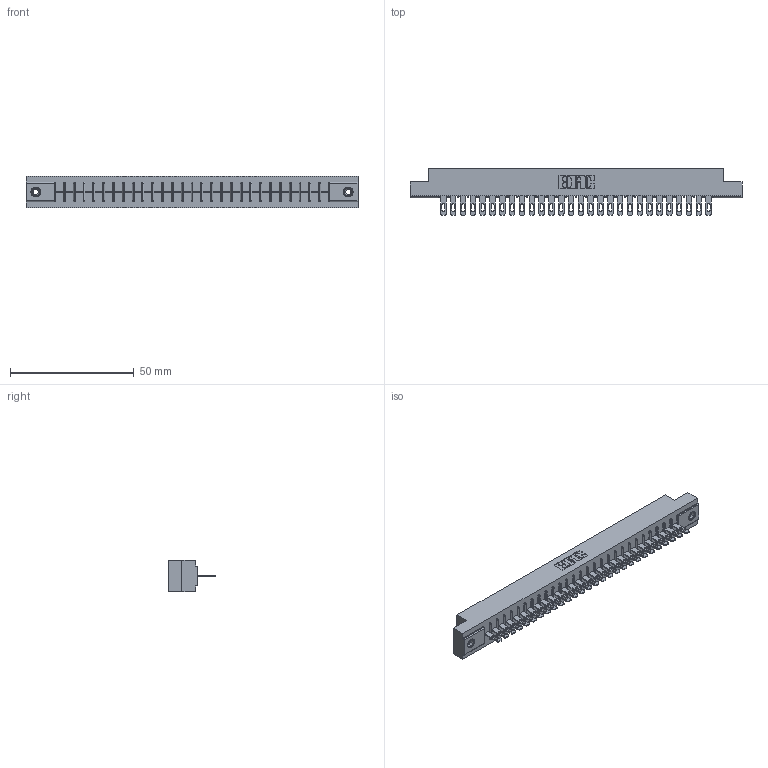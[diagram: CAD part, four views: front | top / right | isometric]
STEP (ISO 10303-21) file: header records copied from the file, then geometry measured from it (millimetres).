
FILE_DESCRIPTION (( 'STEP AP203' ), '1' );
FILE_NAME ('316-028-400-108.STEP', '2020-09-22T23:19:40', ( '' ), ( '' ), 'SwSTEP 2.0', 'SolidWorks 2020', '' );
FILE_SCHEMA (( 'CONFIG_CONTROL_DESIGN' ));
Length unit declared in the file: inch
Products named in the file (4): 345-250-001_345-250-003-102; 306-290-001_100; 316-028-400-108; 306 Part_.156 Dia
Assembly tree (31 placements, depth 2):
  316-028-400-108
    306 Part_.156 Dia
    306-290-001_100  x28
    345-250-001_345-250-003-102  x2
Bounding box: 133.96 x 18.87 x 12.7 mm (x, y, z)
Volume: 14774.8 mm3; surface area: 15519.6 mm2
Topology: 31 solids, 31 shells, 2304 faces, 6472 edges, 4156 vertices
Faces by surface type: plane 1500, cylinder 676, sphere 112, cone 12, torus 4
Entity records: 29274 total; most frequent: CARTESIAN_POINT 4894, ORIENTED_EDGE 4844, DIRECTION 4836, EDGE_CURVE 2422, VECTOR 1884, LINE 1884, VERTEX_POINT 1534, AXIS2_PLACEMENT_3D 1476
